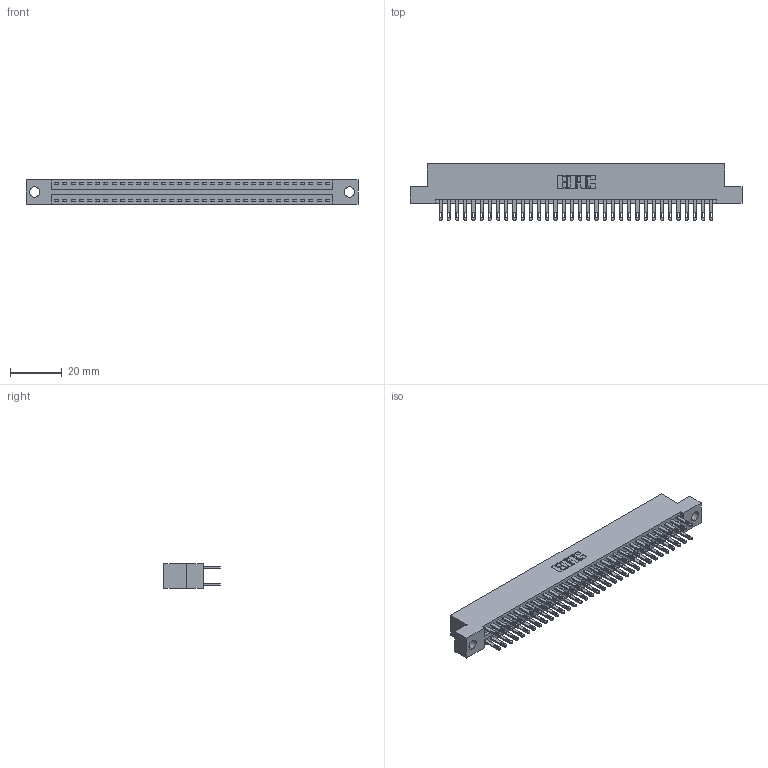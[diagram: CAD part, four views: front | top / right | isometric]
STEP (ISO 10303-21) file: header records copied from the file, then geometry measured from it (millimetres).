
FILE_DESCRIPTION (( 'STEP AP203' ), '1' );
FILE_NAME ('896-068-500-204.STEP', '2021-07-28T01:01:50', ( '' ), ( '' ), 'SwSTEP 2.0', 'SolidWorks 2020', '' );
FILE_SCHEMA (( 'CONFIG_CONTROL_DESIGN' ));
Length unit declared in the file: inch
Products named in the file (3): 846 Part_Flush Mounting Lugs - 0.156 Dia-TH; 345-292-001_345-293-100; 896-068-500-204
Assembly tree (69 placements, depth 2):
  896-068-500-204
    846 Part_Flush Mounting Lugs - 0.156 Dia-TH
    345-292-001_345-293-100  x68
Bounding box: 128.52 x 21.84 x 9.4 mm (x, y, z)
Volume: 12590.5 mm3; surface area: 17705.8 mm2
Topology: 69 solids, 69 shells, 3386 faces, 10325 edges, 6882 vertices
Faces by surface type: plane 2048, cylinder 1338
Entity records: 23199 total; most frequent: CARTESIAN_POINT 3832, ORIENTED_EDGE 3766, DIRECTION 3431, EDGE_CURVE 1883, VECTOR 1611, LINE 1611, VERTEX_POINT 1254, AXIS2_PLACEMENT_3D 910
